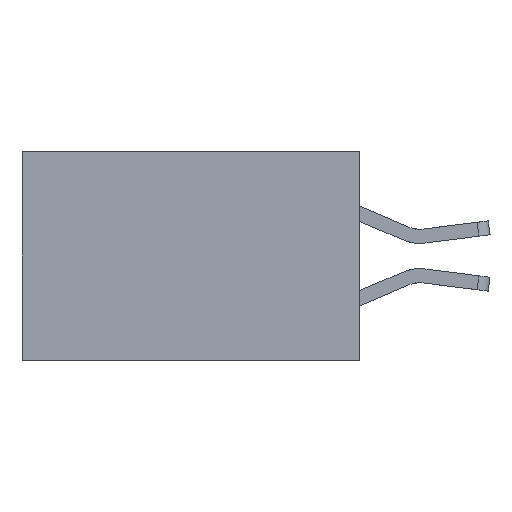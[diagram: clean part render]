
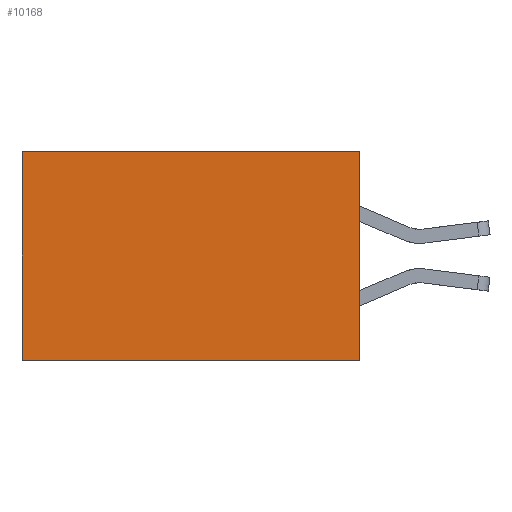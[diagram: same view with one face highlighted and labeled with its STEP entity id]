
A CAD part, left-side view. The second image highlights one B-rep face of the part: STEP entity #10168.
In plain terms, the highlighted planar face has unit normal (-1, 0, 0).
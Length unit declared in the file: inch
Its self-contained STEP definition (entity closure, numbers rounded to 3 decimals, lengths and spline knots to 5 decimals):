
#612 = DIRECTION ( 'NONE',  ( 1., 0., 0. ) ) ;
#712 = VERTEX_POINT ( 'NONE', #12161 ) ;
#1026 = VECTOR ( 'NONE', #3568, 39.37008 ) ;
#1072 = VERTEX_POINT ( 'NONE', #4020 ) ;
#1347 = ORIENTED_EDGE ( 'NONE', *, *, #4163, .T. ) ;
#1437 = CARTESIAN_POINT ( 'NONE',  ( 0.2875, 0., 0. ) ) ;
#1554 = EDGE_CURVE ( 'NONE', #1072, #12499, #5106, .T. ) ;
#2157 = EDGE_LOOP ( 'NONE', ( #1347, #5440, #9878, #2960 ) ) ;
#2474 = EDGE_CURVE ( 'NONE', #712, #10150, #7165, .T. ) ;
#2960 = ORIENTED_EDGE ( 'NONE', *, *, #1554, .T. ) ;
#3427 = FACE_OUTER_BOUND ( 'NONE', #2157, .T. ) ;
#3513 = CARTESIAN_POINT ( 'NONE',  ( 0.2875, 0., 0. ) ) ;
#3568 = DIRECTION ( 'NONE',  ( 0., 0., -1. ) ) ;
#4020 = CARTESIAN_POINT ( 'NONE',  ( 0.2875, 0., 0. ) ) ;
#4137 = DIRECTION ( 'NONE',  ( 0., 1., 0. ) ) ;
#4163 = EDGE_CURVE ( 'NONE', #12499, #10150, #4187, .T. ) ;
#4186 = CARTESIAN_POINT ( 'NONE',  ( 0.2875, 0., -0.37 ) ) ;
#4187 = LINE ( 'NONE', #10004, #9341 ) ;
#4425 = VECTOR ( 'NONE', #4137, 39.37008 ) ;
#5106 = LINE ( 'NONE', #1437, #12829 ) ;
#5440 = ORIENTED_EDGE ( 'NONE', *, *, #2474, .F. ) ;
#5714 = EDGE_CURVE ( 'NONE', #1072, #712, #8977, .T. ) ;
#6154 = PLANE ( 'NONE',  #8265 ) ;
#6162 = DIRECTION ( 'NONE',  ( 0., 1., 0. ) ) ;
#7165 = LINE ( 'NONE', #4186, #4425 ) ;
#8229 = DIRECTION ( 'NONE',  ( 0., 0., -1. ) ) ;
#8265 = AXIS2_PLACEMENT_3D ( 'NONE', #13143, #612, #8229 ) ;
#8977 = LINE ( 'NONE', #3513, #1026 ) ;
#9341 = VECTOR ( 'NONE', #10234, 39.37008 ) ;
#9878 = ORIENTED_EDGE ( 'NONE', *, *, #5714, .F. ) ;
#10004 = CARTESIAN_POINT ( 'NONE',  ( 0.2875, 0.6, 0. ) ) ;
#10150 = VERTEX_POINT ( 'NONE', #11171 ) ;
#10168 = ADVANCED_FACE ( 'NONE', ( #3427 ), #6154, .F. ) ;
#10234 = DIRECTION ( 'NONE',  ( 0., 0., -1. ) ) ;
#11171 = CARTESIAN_POINT ( 'NONE',  ( 0.2875, 0.6, -0.37 ) ) ;
#11722 = CARTESIAN_POINT ( 'NONE',  ( 0.2875, 0.6, 0. ) ) ;
#12161 = CARTESIAN_POINT ( 'NONE',  ( 0.2875, 0., -0.37 ) ) ;
#12499 = VERTEX_POINT ( 'NONE', #11722 ) ;
#12829 = VECTOR ( 'NONE', #6162, 39.37008 ) ;
#13143 = CARTESIAN_POINT ( 'NONE',  ( 0.2875, 0., 0. ) ) ;
